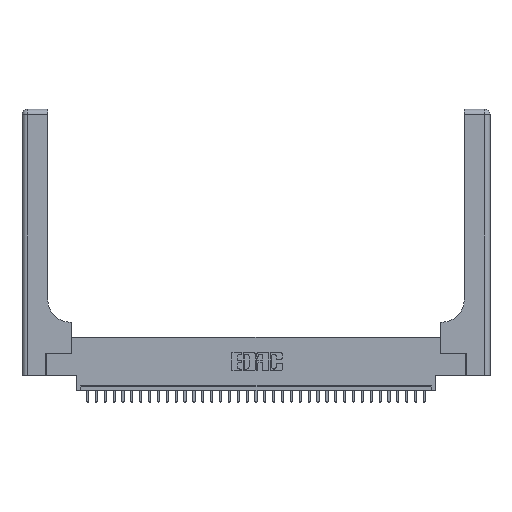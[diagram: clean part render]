
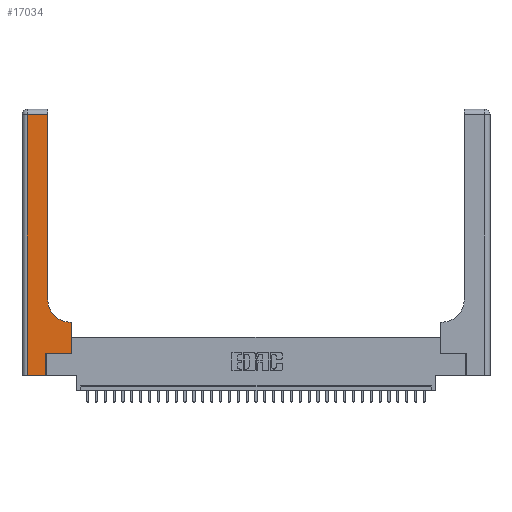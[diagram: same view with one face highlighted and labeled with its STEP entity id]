
A CAD part, top view. The second image highlights one B-rep face of the part: STEP entity #17034.
In plain terms, the highlighted planar face has unit normal (0, 0, 1).
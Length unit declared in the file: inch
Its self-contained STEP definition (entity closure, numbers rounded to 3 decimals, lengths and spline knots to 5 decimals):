
#778 = CARTESIAN_POINT ( 'NONE',  ( 0.2915, 0.85, 0.37 ) ) ;
#1148 = EDGE_CURVE ( 'NONE', #13482, #17894, #8872, .T. ) ;
#1500 = CARTESIAN_POINT ( 'NONE',  ( 0.269, 0., 0.37 ) ) ;
#2420 = DIRECTION ( 'NONE',  ( 0., 1., 0. ) ) ;
#2571 = EDGE_LOOP ( 'NONE', ( #12749, #34141, #25116, #20411, #4918, #29134, #26577, #5722, #14100 ) ) ;
#3854 = LINE ( 'NONE', #6903, #31817 ) ;
#4424 = VERTEX_POINT ( 'NONE', #34337 ) ;
#4693 = EDGE_CURVE ( 'NONE', #34684, #15970, #9361, .T. ) ;
#4918 = ORIENTED_EDGE ( 'NONE', *, *, #7211, .T. ) ;
#5338 = VECTOR ( 'NONE', #28891, 39.37008 ) ;
#5722 = ORIENTED_EDGE ( 'NONE', *, *, #28758, .T. ) ;
#5855 = DIRECTION ( 'NONE',  ( 0., 1., 0. ) ) ;
#6535 = EDGE_CURVE ( 'NONE', #26456, #13482, #7544, .T. ) ;
#6903 = CARTESIAN_POINT ( 'NONE',  ( 0., 2.94, 0.37 ) ) ;
#7211 = EDGE_CURVE ( 'NONE', #4424, #26456, #12101, .T. ) ;
#7268 = VECTOR ( 'NONE', #2420, 39.37008 ) ;
#7544 = LINE ( 'NONE', #17922, #20627 ) ;
#7705 = VERTEX_POINT ( 'NONE', #26021 ) ;
#8866 = LINE ( 'NONE', #21420, #29629 ) ;
#8872 = LINE ( 'NONE', #19798, #7268 ) ;
#9361 = LINE ( 'NONE', #14260, #30486 ) ;
#9641 = DIRECTION ( 'NONE',  ( 1., 0., 0. ) ) ;
#10181 = LINE ( 'NONE', #18318, #13941 ) ;
#11726 = CIRCLE ( 'NONE', #23488, 0.25 ) ;
#12080 = VERTEX_POINT ( 'NONE', #30872 ) ;
#12101 = LINE ( 'NONE', #1500, #5338 ) ;
#12749 = ORIENTED_EDGE ( 'NONE', *, *, #4693, .T. ) ;
#13482 = VERTEX_POINT ( 'NONE', #30286 ) ;
#13941 = VECTOR ( 'NONE', #34444, 39.37008 ) ;
#14100 = ORIENTED_EDGE ( 'NONE', *, *, #26656, .T. ) ;
#14260 = CARTESIAN_POINT ( 'NONE',  ( 0.2915, 3., 0.37 ) ) ;
#14283 = DIRECTION ( 'NONE',  ( 0., 0., -1. ) ) ;
#14539 = DIRECTION ( 'NONE',  ( 0., 0., -1. ) ) ;
#14875 = VECTOR ( 'NONE', #18187, 39.37008 ) ;
#14890 = DIRECTION ( 'NONE',  ( 1., 0., 0. ) ) ;
#15970 = VERTEX_POINT ( 'NONE', #32798 ) ;
#16940 = AXIS2_PLACEMENT_3D ( 'NONE', #27594, #14283, #30859 ) ;
#17034 = ADVANCED_FACE ( 'NONE', ( #31873 ), #17093, .F. ) ;
#17093 = PLANE ( 'NONE',  #16940 ) ;
#17894 = VERTEX_POINT ( 'NONE', #27078 ) ;
#17922 = CARTESIAN_POINT ( 'NONE',  ( 0.269, 0.25, 0.37 ) ) ;
#18187 = DIRECTION ( 'NONE',  ( -1., 0., 0. ) ) ;
#18318 = CARTESIAN_POINT ( 'NONE',  ( 0., 0., 0.37 ) ) ;
#19798 = CARTESIAN_POINT ( 'NONE',  ( 0.5585, 0.25, 0.37 ) ) ;
#20411 = ORIENTED_EDGE ( 'NONE', *, *, #25688, .T. ) ;
#20627 = VECTOR ( 'NONE', #9641, 39.37008 ) ;
#20912 = CARTESIAN_POINT ( 'NONE',  ( 0.269, 0.25, 0.37 ) ) ;
#20965 = DIRECTION ( 'NONE',  ( 0., -1., 0. ) ) ;
#21420 = CARTESIAN_POINT ( 'NONE',  ( 0.06, 3., 0.37 ) ) ;
#23347 = VERTEX_POINT ( 'NONE', #24815 ) ;
#23471 = CARTESIAN_POINT ( 'NONE',  ( 0.2915, 0.6, 0.37 ) ) ;
#23488 = AXIS2_PLACEMENT_3D ( 'NONE', #30749, #14539, #14890 ) ;
#24773 = EDGE_CURVE ( 'NONE', #7705, #23347, #8866, .T. ) ;
#24815 = CARTESIAN_POINT ( 'NONE',  ( 0.06, 0., 0.37 ) ) ;
#25116 = ORIENTED_EDGE ( 'NONE', *, *, #24773, .T. ) ;
#25688 = EDGE_CURVE ( 'NONE', #23347, #4424, #10181, .T. ) ;
#26021 = CARTESIAN_POINT ( 'NONE',  ( 0.06, 2.94, 0.37 ) ) ;
#26456 = VERTEX_POINT ( 'NONE', #20912 ) ;
#26577 = ORIENTED_EDGE ( 'NONE', *, *, #1148, .T. ) ;
#26656 = EDGE_CURVE ( 'NONE', #12080, #34684, #11726, .T. ) ;
#27078 = CARTESIAN_POINT ( 'NONE',  ( 0.5585, 0.6, 0.37 ) ) ;
#27594 = CARTESIAN_POINT ( 'NONE',  ( 0., 3., 0.37 ) ) ;
#28000 = EDGE_CURVE ( 'NONE', #15970, #7705, #3854, .T. ) ;
#28758 = EDGE_CURVE ( 'NONE', #17894, #12080, #32244, .T. ) ;
#28891 = DIRECTION ( 'NONE',  ( 0., 1., 0. ) ) ;
#29134 = ORIENTED_EDGE ( 'NONE', *, *, #6535, .T. ) ;
#29629 = VECTOR ( 'NONE', #20965, 39.37008 ) ;
#30286 = CARTESIAN_POINT ( 'NONE',  ( 0.5585, 0.25, 0.37 ) ) ;
#30486 = VECTOR ( 'NONE', #5855, 39.37008 ) ;
#30749 = CARTESIAN_POINT ( 'NONE',  ( 0.5415, 0.85, 0.37 ) ) ;
#30859 = DIRECTION ( 'NONE',  ( -1., 0., 0. ) ) ;
#30872 = CARTESIAN_POINT ( 'NONE',  ( 0.5415, 0.6, 0.37 ) ) ;
#31817 = VECTOR ( 'NONE', #34009, 39.37008 ) ;
#31873 = FACE_OUTER_BOUND ( 'NONE', #2571, .T. ) ;
#32244 = LINE ( 'NONE', #23471, #14875 ) ;
#32798 = CARTESIAN_POINT ( 'NONE',  ( 0.2915, 2.94, 0.37 ) ) ;
#34009 = DIRECTION ( 'NONE',  ( -1., 0., 0. ) ) ;
#34141 = ORIENTED_EDGE ( 'NONE', *, *, #28000, .T. ) ;
#34337 = CARTESIAN_POINT ( 'NONE',  ( 0.269, 0., 0.37 ) ) ;
#34444 = DIRECTION ( 'NONE',  ( 1., 0., 0. ) ) ;
#34684 = VERTEX_POINT ( 'NONE', #778 ) ;
